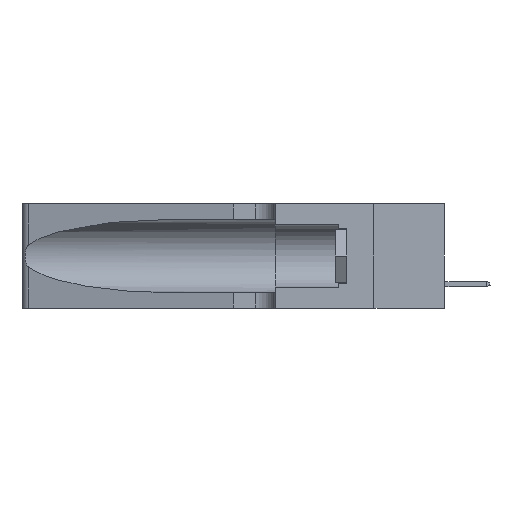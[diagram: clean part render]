
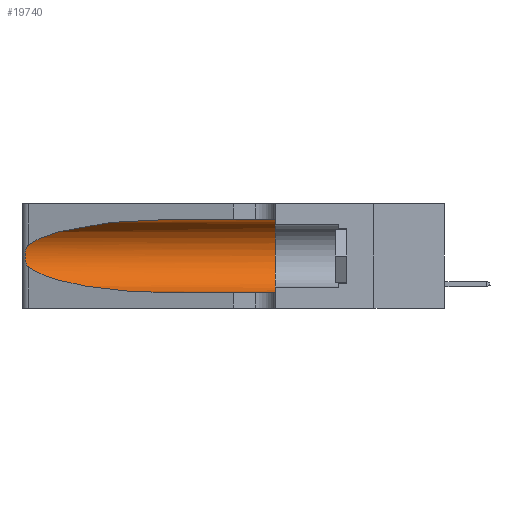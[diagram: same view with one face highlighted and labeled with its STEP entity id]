
A CAD part, left-side view. The second image highlights one B-rep face of the part: STEP entity #19740.
In plain terms, the highlighted cylindrical face has radius 3.308 mm (diameter 6.617 mm), a partial arc.
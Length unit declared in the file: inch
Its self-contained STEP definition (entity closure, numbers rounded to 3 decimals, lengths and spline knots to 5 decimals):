
#109 = CARTESIAN_POINT ( 'NONE',  ( 0.1305, 1.61858, 0.185 ) ) ;
#211 = ORIENTED_EDGE ( 'NONE', *, *, #15243, .T. ) ;
#315 = CARTESIAN_POINT ( 'NONE',  ( 0.25487, 1.22718, 0.14631 ) ) ;
#818 = CARTESIAN_POINT ( 'NONE',  ( 0.25487, 1.22718, 0.22369 ) ) ;
#929 = LINE ( 'NONE', #5587, #4018 ) ;
#969 = AXIS2_PLACEMENT_3D ( 'NONE', #109, #10081, #8630 ) ;
#1029 = ORIENTED_EDGE ( 'NONE', *, *, #15491, .T. ) ;
#1336 = CARTESIAN_POINT ( 'NONE',  ( 0.1305, 0.72297, 0.05475 ) ) ;
#1562 = VERTEX_POINT ( 'NONE', #11947 ) ;
#1594 = CARTESIAN_POINT ( 'NONE',  ( 0.25854, 1.2359, 0.20912 ) ) ;
#1751 = CARTESIAN_POINT ( 'NONE',  ( 0.26075, 1.23896, 0.178 ) ) ;
#2126 = VERTEX_POINT ( 'NONE', #6504 ) ;
#2964 = VERTEX_POINT ( 'NONE', #818 ) ;
#4018 = VECTOR ( 'NONE', #17260, 39.37008 ) ;
#4119 = CIRCLE ( 'NONE', #21251, 0.13025 ) ;
#4271 = CARTESIAN_POINT ( 'NONE',  ( 0.1305, 0.72297, 0.05475 ) ) ;
#4944 = CARTESIAN_POINT ( 'NONE',  ( 0.18966, 0.96281, 0.31525 ) ) ;
#4987 = CARTESIAN_POINT ( 'NONE',  ( 0.25639, 1.23184, 0.21858 ) ) ;
#5141 = CARTESIAN_POINT ( 'NONE',  ( 0.25787, 1.23484, 0.2124 ) ) ;
#5220 = CARTESIAN_POINT ( 'NONE',  ( 0.25639, 1.23186, 0.15144 ) ) ;
#5383 = B_SPLINE_CURVE_WITH_KNOTS ( 'NONE', 3,
 ( #9814, #11514, #4987, #5141, #1594, #6658, #8302, #1751, #15009, #10050, #11735, #5220, #8530, #17040 ),
 .UNSPECIFIED., .F., .F.,
 ( 4, 2, 2, 2, 2, 2, 4 ),
 ( 0., 0.00027, 0.00053, 0.00107, 0.0016, 0.00187, 0.00214 ),
 .UNSPECIFIED. ) ;
#5587 = CARTESIAN_POINT ( 'NONE',  ( 0.1305, 1.61858, 0.05475 ) ) ;
#6001 = EDGE_CURVE ( 'NONE', #12801, #1562, #20798, .T. ) ;
#6504 = CARTESIAN_POINT ( 'NONE',  ( 0.25487, 1.22718, 0.14631 ) ) ;
#6658 = CARTESIAN_POINT ( 'NONE',  ( 0.26018, 1.23835, 0.19895 ) ) ;
#7626 = EDGE_CURVE ( 'NONE', #1562, #19196, #4119, .T. ) ;
#8302 = CARTESIAN_POINT ( 'NONE',  ( 0.26075, 1.23896, 0.19203 ) ) ;
#8530 = CARTESIAN_POINT ( 'NONE',  ( 0.25555, 1.22993, 0.14849 ) ) ;
#8630 = DIRECTION ( 'NONE',  ( 0., 0., -1. ) ) ;
#8681 = CARTESIAN_POINT ( 'NONE',  ( 0.2373, 1.15595, 0.08982 ) ) ;
#9236 = VERTEX_POINT ( 'NONE', #1336 ) ;
#9584 =( BOUNDED_CURVE ( )  B_SPLINE_CURVE ( 3, ( #315, #8681, #14133, #4271 ),
 .UNSPECIFIED., .F., .F. ) 
 B_SPLINE_CURVE_WITH_KNOTS ( ( 4, 4 ),
 ( 3.44316, 4.71239 ),
 .UNSPECIFIED. ) 
 CURVE ( )  GEOMETRIC_REPRESENTATION_ITEM ( )  RATIONAL_B_SPLINE_CURVE ( ( 1., 0.87, 0.87, 1. ) ) 
 REPRESENTATION_ITEM ( '' )  );
#9814 = CARTESIAN_POINT ( 'NONE',  ( 0.25487, 1.22718, 0.22369 ) ) ;
#10050 = CARTESIAN_POINT ( 'NONE',  ( 0.25856, 1.23593, 0.16098 ) ) ;
#10081 = DIRECTION ( 'NONE',  ( 0., -1., 0. ) ) ;
#11007 = CARTESIAN_POINT ( 'NONE',  ( 0.1305, 0.72297, 0.31525 ) ) ;
#11514 = CARTESIAN_POINT ( 'NONE',  ( 0.25555, 1.22994, 0.2215 ) ) ;
#11735 = CARTESIAN_POINT ( 'NONE',  ( 0.25789, 1.23486, 0.15765 ) ) ;
#11832 = CARTESIAN_POINT ( 'NONE',  ( 0.1305, 0.72297, 0.31525 ) ) ;
#11947 = CARTESIAN_POINT ( 'NONE',  ( 0.1305, 0.35, 0.31525 ) ) ;
#12081 = CARTESIAN_POINT ( 'NONE',  ( 0.1305, 0.35, 0.185 ) ) ;
#12092 = EDGE_CURVE ( 'NONE', #2964, #2126, #5383, .T. ) ;
#12283 = FACE_OUTER_BOUND ( 'NONE', #13953, .T. ) ;
#12646 = ORIENTED_EDGE ( 'NONE', *, *, #7626, .F. ) ;
#12801 = VERTEX_POINT ( 'NONE', #11007 ) ;
#13493 =( BOUNDED_CURVE ( )  B_SPLINE_CURVE ( 3, ( #11832, #4944, #15271, #16848 ),
 .UNSPECIFIED., .F., .T. ) 
 B_SPLINE_CURVE_WITH_KNOTS ( ( 4, 4 ),
 ( 1.5708, 2.84003 ),
 .UNSPECIFIED. ) 
 CURVE ( )  GEOMETRIC_REPRESENTATION_ITEM ( )  RATIONAL_B_SPLINE_CURVE ( ( 1., 0.87, 0.87, 1. ) ) 
 REPRESENTATION_ITEM ( '' )  );
#13821 = EDGE_CURVE ( 'NONE', #12801, #2964, #13493, .T. ) ;
#13953 = EDGE_LOOP ( 'NONE', ( #14616, #17531, #211, #1029, #12646, #14157 ) ) ;
#13976 = DIRECTION ( 'NONE',  ( 0., 0., 1. ) ) ;
#14133 = CARTESIAN_POINT ( 'NONE',  ( 0.18966, 0.96281, 0.05475 ) ) ;
#14157 = ORIENTED_EDGE ( 'NONE', *, *, #6001, .F. ) ;
#14249 = DIRECTION ( 'NONE',  ( 0., 1., 0. ) ) ;
#14262 = VECTOR ( 'NONE', #14289, 39.37008 ) ;
#14289 = DIRECTION ( 'NONE',  ( 0., -1., 0. ) ) ;
#14616 = ORIENTED_EDGE ( 'NONE', *, *, #13821, .T. ) ;
#15009 = CARTESIAN_POINT ( 'NONE',  ( 0.26017, 1.23833, 0.17102 ) ) ;
#15243 = EDGE_CURVE ( 'NONE', #2126, #9236, #9584, .T. ) ;
#15271 = CARTESIAN_POINT ( 'NONE',  ( 0.2373, 1.15595, 0.28018 ) ) ;
#15491 = EDGE_CURVE ( 'NONE', #9236, #19196, #929, .T. ) ;
#16848 = CARTESIAN_POINT ( 'NONE',  ( 0.25487, 1.22718, 0.22369 ) ) ;
#17040 = CARTESIAN_POINT ( 'NONE',  ( 0.25487, 1.22718, 0.14631 ) ) ;
#17260 = DIRECTION ( 'NONE',  ( 0., -1., 0. ) ) ;
#17531 = ORIENTED_EDGE ( 'NONE', *, *, #12092, .T. ) ;
#18319 = CARTESIAN_POINT ( 'NONE',  ( 0.1305, 0.35, 0.05475 ) ) ;
#19196 = VERTEX_POINT ( 'NONE', #18319 ) ;
#19329 = CARTESIAN_POINT ( 'NONE',  ( 0.1305, 1.61858, 0.31525 ) ) ;
#19740 = ADVANCED_FACE ( 'NONE', ( #12283 ), #20081, .F. ) ;
#20081 = CYLINDRICAL_SURFACE ( 'NONE', #969, 0.13025 ) ;
#20798 = LINE ( 'NONE', #19329, #14262 ) ;
#21251 = AXIS2_PLACEMENT_3D ( 'NONE', #12081, #14249, #13976 ) ;
